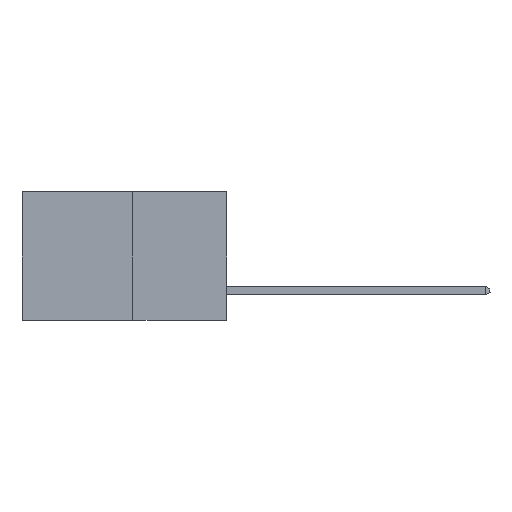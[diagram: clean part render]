
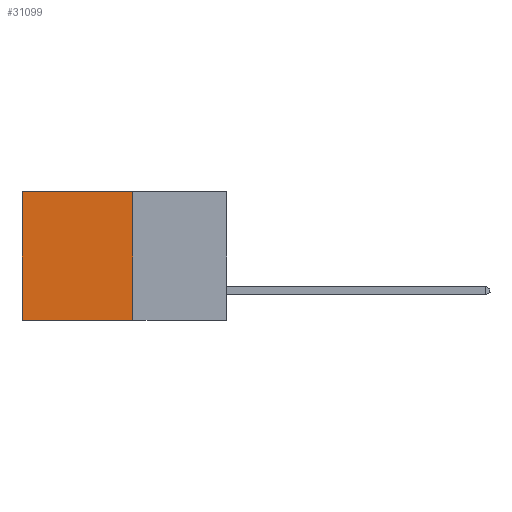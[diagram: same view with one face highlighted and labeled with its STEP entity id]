
A CAD part, left-side view. The second image highlights one B-rep face of the part: STEP entity #31099.
In plain terms, the highlighted planar face has unit normal (-1, 0, 0).
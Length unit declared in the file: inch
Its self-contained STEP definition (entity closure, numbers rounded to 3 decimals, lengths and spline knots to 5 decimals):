
#907 = ORIENTED_EDGE ( 'NONE', *, *, #19623, .F. ) ;
#1150 = CARTESIAN_POINT ( 'NONE',  ( 0.277, 0.27, -0.37 ) ) ;
#1199 = FACE_OUTER_BOUND ( 'NONE', #19111, .T. ) ;
#3643 = CARTESIAN_POINT ( 'NONE',  ( 0.277, 0.27, 0. ) ) ;
#4173 = EDGE_CURVE ( 'NONE', #22057, #8123, #24741, .T. ) ;
#5339 = VECTOR ( 'NONE', #30632, 39.37008 ) ;
#5444 = VECTOR ( 'NONE', #24732, 39.37008 ) ;
#6239 = LINE ( 'NONE', #26355, #24030 ) ;
#6453 = DIRECTION ( 'NONE',  ( 0., 0., -1. ) ) ;
#8123 = VERTEX_POINT ( 'NONE', #14617 ) ;
#8614 = VERTEX_POINT ( 'NONE', #30960 ) ;
#9413 = EDGE_CURVE ( 'NONE', #8614, #8123, #6239, .T. ) ;
#13394 = ORIENTED_EDGE ( 'NONE', *, *, #4173, .F. ) ;
#14617 = CARTESIAN_POINT ( 'NONE',  ( 0.277, 0.59, -0.37 ) ) ;
#16315 = EDGE_CURVE ( 'NONE', #20069, #8614, #23867, .T. ) ;
#17142 = CARTESIAN_POINT ( 'NONE',  ( 0.277, 0.27, -0.37 ) ) ;
#17162 = VECTOR ( 'NONE', #21181, 39.37008 ) ;
#18480 = ORIENTED_EDGE ( 'NONE', *, *, #9413, .T. ) ;
#18812 = AXIS2_PLACEMENT_3D ( 'NONE', #1150, #21574, #6453 ) ;
#18921 = LINE ( 'NONE', #17142, #5444 ) ;
#18926 = PLANE ( 'NONE',  #18812 ) ;
#18944 = DIRECTION ( 'NONE',  ( 0., 0., -1. ) ) ;
#19111 = EDGE_LOOP ( 'NONE', ( #18480, #13394, #907, #24244 ) ) ;
#19623 = EDGE_CURVE ( 'NONE', #20069, #22057, #18921, .T. ) ;
#20069 = VERTEX_POINT ( 'NONE', #3643 ) ;
#21181 = DIRECTION ( 'NONE',  ( 0., 1., 0. ) ) ;
#21574 = DIRECTION ( 'NONE',  ( 1., 0., 0. ) ) ;
#22057 = VERTEX_POINT ( 'NONE', #23903 ) ;
#23867 = LINE ( 'NONE', #28731, #17162 ) ;
#23903 = CARTESIAN_POINT ( 'NONE',  ( 0.277, 0.27, -0.37 ) ) ;
#24030 = VECTOR ( 'NONE', #18944, 39.37008 ) ;
#24244 = ORIENTED_EDGE ( 'NONE', *, *, #16315, .T. ) ;
#24732 = DIRECTION ( 'NONE',  ( 0., 0., -1. ) ) ;
#24741 = LINE ( 'NONE', #30454, #5339 ) ;
#26355 = CARTESIAN_POINT ( 'NONE',  ( 0.277, 0.59, -0.37 ) ) ;
#28731 = CARTESIAN_POINT ( 'NONE',  ( 0.277, 0.27, 0. ) ) ;
#30454 = CARTESIAN_POINT ( 'NONE',  ( 0.277, 0.27, -0.37 ) ) ;
#30632 = DIRECTION ( 'NONE',  ( 0., 1., 0. ) ) ;
#30960 = CARTESIAN_POINT ( 'NONE',  ( 0.277, 0.59, 0. ) ) ;
#31099 = ADVANCED_FACE ( 'NONE', ( #1199 ), #18926, .F. ) ;
